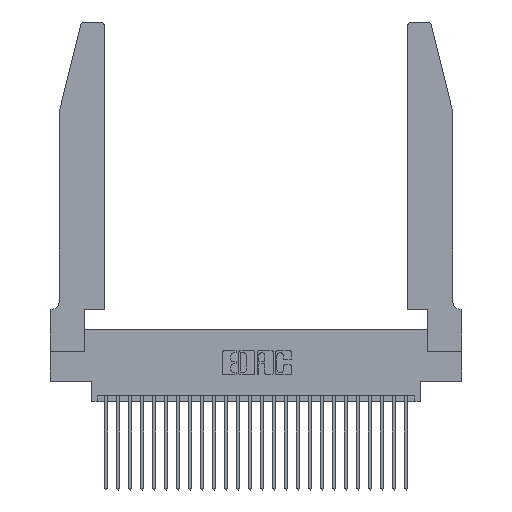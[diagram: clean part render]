
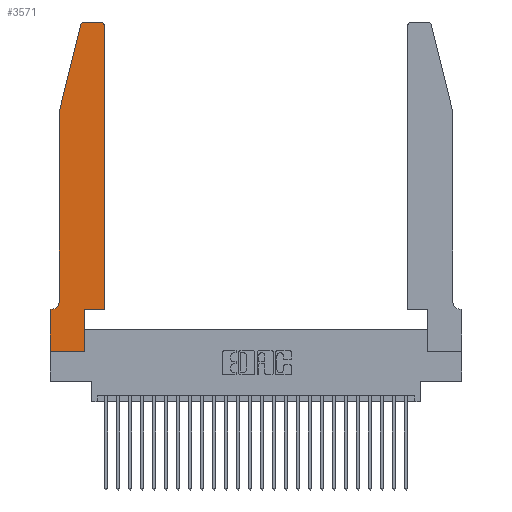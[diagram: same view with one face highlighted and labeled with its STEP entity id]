
A CAD part, top view. The second image highlights one B-rep face of the part: STEP entity #3571.
In plain terms, the highlighted planar face has unit normal (0, 0, 1).
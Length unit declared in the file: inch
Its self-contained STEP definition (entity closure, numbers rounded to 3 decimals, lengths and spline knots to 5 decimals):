
#248 = EDGE_CURVE ( 'NONE', #1336, #21746, #6291, .T. ) ;
#417 = LINE ( 'NONE', #3408, #11320 ) ;
#512 = ORIENTED_EDGE ( 'NONE', *, *, #27228, .T. ) ;
#658 = DIRECTION ( 'NONE',  ( 0., -1., 0. ) ) ;
#741 = CARTESIAN_POINT ( 'NONE',  ( 0.0755, 0.35, 0.37 ) ) ;
#1077 = CARTESIAN_POINT ( 'NONE',  ( 0., 0.35, 0.37 ) ) ;
#1230 = LINE ( 'NONE', #10245, #17712 ) ;
#1232 = DIRECTION ( 'NONE',  ( 0., 1., 0. ) ) ;
#1336 = VERTEX_POINT ( 'NONE', #3776 ) ;
#2188 = VERTEX_POINT ( 'NONE', #11751 ) ;
#2307 = ORIENTED_EDGE ( 'NONE', *, *, #17387, .T. ) ;
#2519 = ORIENTED_EDGE ( 'NONE', *, *, #24019, .T. ) ;
#2790 = CARTESIAN_POINT ( 'NONE',  ( 0.0755, 2., 0.37 ) ) ;
#2824 = ORIENTED_EDGE ( 'NONE', *, *, #4859, .T. ) ;
#2955 = DIRECTION ( 'NONE',  ( 0., 0., -1. ) ) ;
#2973 = DIRECTION ( 'NONE',  ( -1., 0., 0. ) ) ;
#3062 = CARTESIAN_POINT ( 'NONE',  ( 0.0055, 0.35, 0.37 ) ) ;
#3408 = CARTESIAN_POINT ( 'NONE',  ( 0.0755, 2., 0.37 ) ) ;
#3561 = FACE_OUTER_BOUND ( 'NONE', #13386, .T. ) ;
#3571 = ADVANCED_FACE ( 'NONE', ( #3561 ), #7329, .T. ) ;
#3610 = CIRCLE ( 'NONE', #26144, 0.03 ) ;
#3776 = CARTESIAN_POINT ( 'NONE',  ( 0.2865, 0.35, 0.37 ) ) ;
#3877 = CARTESIAN_POINT ( 'NONE',  ( 0.0755, 2., 0.37 ) ) ;
#4020 = AXIS2_PLACEMENT_3D ( 'NONE', #21704, #9078, #23784 ) ;
#4300 = CARTESIAN_POINT ( 'NONE',  ( 0.25487, 2.72718, 0.37 ) ) ;
#4332 = VERTEX_POINT ( 'NONE', #3877 ) ;
#4523 = CARTESIAN_POINT ( 'NONE',  ( 0.284, 2.75, 0.37 ) ) ;
#4859 = EDGE_CURVE ( 'NONE', #21746, #15243, #13619, .T. ) ;
#5459 = AXIS2_PLACEMENT_3D ( 'NONE', #15849, #2955, #17930 ) ;
#5567 = ORIENTED_EDGE ( 'NONE', *, *, #17214, .T. ) ;
#5582 = DIRECTION ( 'NONE',  ( -0.239, -0.971, 0. ) ) ;
#6291 = LINE ( 'NONE', #12156, #16980 ) ;
#6473 = LINE ( 'NONE', #2790, #17802 ) ;
#6512 = EDGE_CURVE ( 'NONE', #15243, #20033, #19805, .T. ) ;
#6783 = LINE ( 'NONE', #10278, #17473 ) ;
#7081 = VECTOR ( 'NONE', #2973, 39.37008 ) ;
#7329 = PLANE ( 'NONE',  #18821 ) ;
#7425 = DIRECTION ( 'NONE',  ( 1., 0., 0. ) ) ;
#7450 = ORIENTED_EDGE ( 'NONE', *, *, #24126, .T. ) ;
#7589 = VERTEX_POINT ( 'NONE', #1077 ) ;
#8587 = VECTOR ( 'NONE', #1232, 39.37008 ) ;
#8934 = CARTESIAN_POINT ( 'NONE',  ( 0.284, 2.72, 0.37 ) ) ;
#8971 = DIRECTION ( 'NONE',  ( 0., 1., 0. ) ) ;
#9078 = DIRECTION ( 'NONE',  ( 0., 0., 1. ) ) ;
#9087 = EDGE_CURVE ( 'NONE', #7589, #16040, #1230, .T. ) ;
#9192 = ORIENTED_EDGE ( 'NONE', *, *, #20102, .T. ) ;
#9806 = VERTEX_POINT ( 'NONE', #4523 ) ;
#10245 = CARTESIAN_POINT ( 'NONE',  ( 0., 0., 0.37 ) ) ;
#10278 = CARTESIAN_POINT ( 'NONE',  ( 0., 0., 0.37 ) ) ;
#10282 = VERTEX_POINT ( 'NONE', #4300 ) ;
#11090 = DIRECTION ( 'NONE',  ( 1., 0., 0. ) ) ;
#11320 = VECTOR ( 'NONE', #5582, 39.37008 ) ;
#11751 = CARTESIAN_POINT ( 'NONE',  ( 0.0755, 0.42, 0.37 ) ) ;
#12156 = CARTESIAN_POINT ( 'NONE',  ( 0.4505, 0.35, 0.37 ) ) ;
#12434 = DIRECTION ( 'NONE',  ( 1., 0., 0. ) ) ;
#12626 = DIRECTION ( 'NONE',  ( 1., 0., 0. ) ) ;
#12858 = VECTOR ( 'NONE', #12913, 39.37008 ) ;
#12913 = DIRECTION ( 'NONE',  ( -1., 0., 0. ) ) ;
#13386 = EDGE_LOOP ( 'NONE', ( #2307, #512, #21376, #7450, #9192, #27313, #24255, #5567, #2519, #15190, #2824, #13445 ) ) ;
#13445 = ORIENTED_EDGE ( 'NONE', *, *, #6512, .T. ) ;
#13619 = LINE ( 'NONE', #16318, #8587 ) ;
#14199 = VECTOR ( 'NONE', #8971, 39.37008 ) ;
#14244 = VERTEX_POINT ( 'NONE', #3062 ) ;
#15190 = ORIENTED_EDGE ( 'NONE', *, *, #248, .T. ) ;
#15243 = VERTEX_POINT ( 'NONE', #23154 ) ;
#15849 = CARTESIAN_POINT ( 'NONE',  ( 0.0055, 0.42, 0.37 ) ) ;
#15956 = CARTESIAN_POINT ( 'NONE',  ( 0., 0.35, 0.37 ) ) ;
#16040 = VERTEX_POINT ( 'NONE', #21046 ) ;
#16318 = CARTESIAN_POINT ( 'NONE',  ( 0.4505, 0.35, 0.37 ) ) ;
#16980 = VECTOR ( 'NONE', #12626, 39.37008 ) ;
#17214 = EDGE_CURVE ( 'NONE', #16040, #18758, #6783, .T. ) ;
#17387 = EDGE_CURVE ( 'NONE', #20033, #9806, #18425, .T. ) ;
#17473 = VECTOR ( 'NONE', #12434, 39.37008 ) ;
#17660 = CARTESIAN_POINT ( 'NONE',  ( 0.4205, 2.75, 0.37 ) ) ;
#17712 = VECTOR ( 'NONE', #22800, 39.37008 ) ;
#17802 = VECTOR ( 'NONE', #658, 39.37008 ) ;
#17930 = DIRECTION ( 'NONE',  ( -1., 0., 0. ) ) ;
#18402 = LINE ( 'NONE', #741, #7081 ) ;
#18425 = LINE ( 'NONE', #23314, #12858 ) ;
#18758 = VERTEX_POINT ( 'NONE', #23734 ) ;
#18821 = AXIS2_PLACEMENT_3D ( 'NONE', #15956, #20161, #7425 ) ;
#19789 = LINE ( 'NONE', #25736, #14199 ) ;
#19805 = CIRCLE ( 'NONE', #4020, 0.03 ) ;
#20033 = VERTEX_POINT ( 'NONE', #17660 ) ;
#20102 = EDGE_CURVE ( 'NONE', #2188, #14244, #26993, .T. ) ;
#20161 = DIRECTION ( 'NONE',  ( 0., 0., 1. ) ) ;
#20770 = EDGE_CURVE ( 'NONE', #10282, #4332, #417, .T. ) ;
#21046 = CARTESIAN_POINT ( 'NONE',  ( 0., 0., 0.37 ) ) ;
#21376 = ORIENTED_EDGE ( 'NONE', *, *, #20770, .T. ) ;
#21704 = CARTESIAN_POINT ( 'NONE',  ( 0.4205, 2.72, 0.37 ) ) ;
#21746 = VERTEX_POINT ( 'NONE', #22324 ) ;
#22324 = CARTESIAN_POINT ( 'NONE',  ( 0.4505, 0.35, 0.37 ) ) ;
#22800 = DIRECTION ( 'NONE',  ( 0., -1., 0. ) ) ;
#23154 = CARTESIAN_POINT ( 'NONE',  ( 0.4505, 2.72, 0.37 ) ) ;
#23314 = CARTESIAN_POINT ( 'NONE',  ( 0.2605, 2.75, 0.37 ) ) ;
#23648 = DIRECTION ( 'NONE',  ( 0., 0., 1. ) ) ;
#23734 = CARTESIAN_POINT ( 'NONE',  ( 0.2865, 0., 0.37 ) ) ;
#23784 = DIRECTION ( 'NONE',  ( 1., 0., 0. ) ) ;
#24019 = EDGE_CURVE ( 'NONE', #18758, #1336, #19789, .T. ) ;
#24126 = EDGE_CURVE ( 'NONE', #4332, #2188, #6473, .T. ) ;
#24255 = ORIENTED_EDGE ( 'NONE', *, *, #9087, .T. ) ;
#24955 = EDGE_CURVE ( 'NONE', #14244, #7589, #18402, .T. ) ;
#25736 = CARTESIAN_POINT ( 'NONE',  ( 0.2865, 0.35, 0.37 ) ) ;
#26144 = AXIS2_PLACEMENT_3D ( 'NONE', #8934, #23648, #11090 ) ;
#26993 = CIRCLE ( 'NONE', #5459, 0.07 ) ;
#27228 = EDGE_CURVE ( 'NONE', #9806, #10282, #3610, .T. ) ;
#27313 = ORIENTED_EDGE ( 'NONE', *, *, #24955, .T. ) ;
